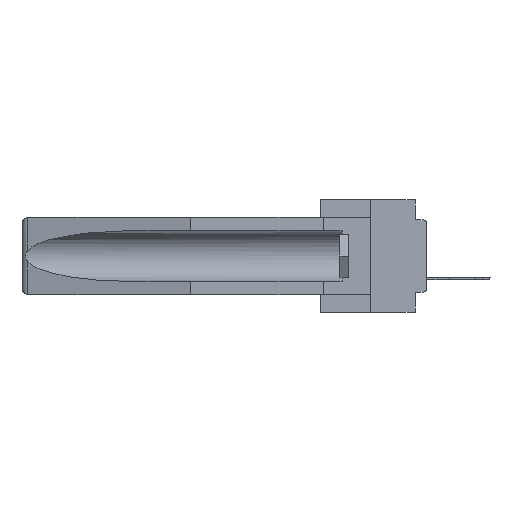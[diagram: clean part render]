
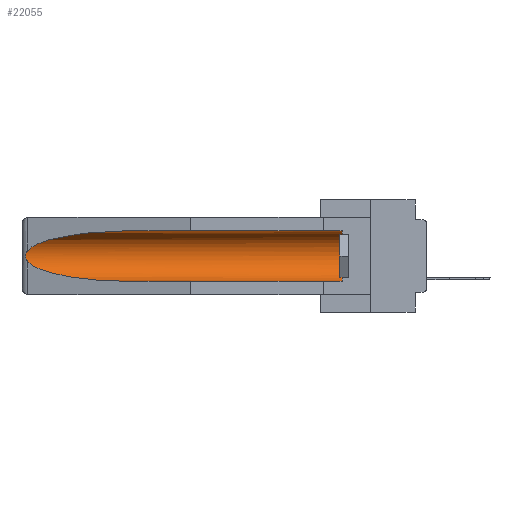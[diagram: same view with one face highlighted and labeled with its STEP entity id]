
A CAD part, left-side view. The second image highlights one B-rep face of the part: STEP entity #22055.
In plain terms, the highlighted cylindrical face has radius 2.857 mm (diameter 5.715 mm), a partial arc.
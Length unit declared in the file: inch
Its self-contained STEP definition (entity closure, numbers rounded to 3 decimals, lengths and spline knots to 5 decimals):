
#254 = CARTESIAN_POINT ( 'NONE',  ( 0.2673, 1.53269, -0.17917 ) ) ;
#654 = CARTESIAN_POINT ( 'NONE',  ( 0.155, 0.126, -0.1715 ) ) ;
#668 = CARTESIAN_POINT ( 'NONE',  ( 0.26537, 1.52718, -0.14972 ) ) ;
#1073 = ORIENTED_EDGE ( 'NONE', *, *, #18933, .F. ) ;
#1545 = LINE ( 'NONE', #14667, #8756 ) ;
#1700 = DIRECTION ( 'NONE',  ( 0., 1., 0. ) ) ;
#3246 = CARTESIAN_POINT ( 'NONE',  ( 0.155, -0.30754, -0.284 ) ) ;
#3362 = FACE_OUTER_BOUND ( 'NONE', #4756, .T. ) ;
#4249 = CARTESIAN_POINT ( 'NONE',  ( 0.26655, 1.53094, -0.18657 ) ) ;
#4392 = CARTESIAN_POINT ( 'NONE',  ( 0.26654, 1.53092, -0.15636 ) ) ;
#4756 = EDGE_LOOP ( 'NONE', ( #9486, #28176, #26582, #1073, #17301, #28006 ) ) ;
#4899 = EDGE_CURVE ( 'NONE', #9115, #27358, #9374, .T. ) ;
#4945 = EDGE_CURVE ( 'NONE', #11408, #9115, #16770, .T. ) ;
#6420 = DIRECTION ( 'NONE',  ( 0., 0., 1. ) ) ;
#7670 = LINE ( 'NONE', #3246, #9727 ) ;
#7814 = DIRECTION ( 'NONE',  ( 0., 1., 0. ) ) ;
#8195 = VERTEX_POINT ( 'NONE', #13341 ) ;
#8678 = CARTESIAN_POINT ( 'NONE',  ( 0.26597, 1.52961, -0.15275 ) ) ;
#8756 = VECTOR ( 'NONE', #1700, 39.37008 ) ;
#8793 = EDGE_CURVE ( 'NONE', #8195, #11408, #1545, .T. ) ;
#8954 = CARTESIAN_POINT ( 'NONE',  ( 0.26537, 1.52718, -0.19328 ) ) ;
#9115 = VERTEX_POINT ( 'NONE', #9651 ) ;
#9374 = B_SPLINE_CURVE_WITH_KNOTS ( 'NONE', 3,
 ( #15514, #8678, #4392, #17663, #15385, #15655, #254, #4249, #11243, #8954 ),
 .UNSPECIFIED., .F., .F.,
 ( 4, 2, 2, 2, 4 ),
 ( 0., 0.00029, 0.00058, 0.00087, 0.00117 ),
 .UNSPECIFIED. ) ;
#9486 = ORIENTED_EDGE ( 'NONE', *, *, #4945, .T. ) ;
#9496 = DIRECTION ( 'NONE',  ( 0., -1., 0. ) ) ;
#9651 = CARTESIAN_POINT ( 'NONE',  ( 0.26537, 1.52718, -0.14972 ) ) ;
#9652 = CARTESIAN_POINT ( 'NONE',  ( 0.155, -0.30754, -0.1715 ) ) ;
#9727 = VECTOR ( 'NONE', #7814, 39.37008 ) ;
#11243 = CARTESIAN_POINT ( 'NONE',  ( 0.26597, 1.5296, -0.19026 ) ) ;
#11408 = VERTEX_POINT ( 'NONE', #16053 ) ;
#11483 = EDGE_CURVE ( 'NONE', #27839, #8195, #13899, .T. ) ;
#11609 = CARTESIAN_POINT ( 'NONE',  ( 0.155, 0.126, -0.284 ) ) ;
#12072 = DIRECTION ( 'NONE',  ( 0., 1., 0. ) ) ;
#12428 = CARTESIAN_POINT ( 'NONE',  ( 0.26537, 1.52718, -0.19328 ) ) ;
#13341 = CARTESIAN_POINT ( 'NONE',  ( 0.155, 0.126, -0.059 ) ) ;
#13457 = AXIS2_PLACEMENT_3D ( 'NONE', #9652, #12072, #20755 ) ;
#13861 = CARTESIAN_POINT ( 'NONE',  ( 0.155, 1.07973, -0.284 ) ) ;
#13899 = CIRCLE ( 'NONE', #27975, 0.1125 ) ;
#14030 =( BOUNDED_CURVE ( )  B_SPLINE_CURVE ( 3, ( #26724, #21908, #17021, #15174 ),
 .UNSPECIFIED., .F., .F. ) 
 B_SPLINE_CURVE_WITH_KNOTS ( ( 4, 4 ),
 ( 0.1948, 1.5708 ),
 .UNSPECIFIED. ) 
 CURVE ( )  GEOMETRIC_REPRESENTATION_ITEM ( )  RATIONAL_B_SPLINE_CURVE ( ( 1., 0.848, 0.848, 1. ) ) 
 REPRESENTATION_ITEM ( '' )  );
#14070 = CARTESIAN_POINT ( 'NONE',  ( 0.155, 1.07973, -0.059 ) ) ;
#14667 = CARTESIAN_POINT ( 'NONE',  ( 0.155, -0.30754, -0.059 ) ) ;
#15174 = CARTESIAN_POINT ( 'NONE',  ( 0.155, 1.07973, -0.284 ) ) ;
#15385 = CARTESIAN_POINT ( 'NONE',  ( 0.2675, 1.53308, -0.16763 ) ) ;
#15514 = CARTESIAN_POINT ( 'NONE',  ( 0.26537, 1.52718, -0.14972 ) ) ;
#15655 = CARTESIAN_POINT ( 'NONE',  ( 0.2675, 1.53308, -0.17534 ) ) ;
#16053 = CARTESIAN_POINT ( 'NONE',  ( 0.155, 1.07973, -0.059 ) ) ;
#16770 =( BOUNDED_CURVE ( )  B_SPLINE_CURVE ( 3, ( #14070, #22329, #18074, #668 ),
 .UNSPECIFIED., .F., .F. ) 
 B_SPLINE_CURVE_WITH_KNOTS ( ( 4, 4 ),
 ( 4.71239, 6.08839 ),
 .UNSPECIFIED. ) 
 CURVE ( )  GEOMETRIC_REPRESENTATION_ITEM ( )  RATIONAL_B_SPLINE_CURVE ( ( 1., 0.848, 0.848, 1. ) ) 
 REPRESENTATION_ITEM ( '' )  );
#17021 = CARTESIAN_POINT ( 'NONE',  ( 0.21114, 1.30732, -0.284 ) ) ;
#17301 = ORIENTED_EDGE ( 'NONE', *, *, #11483, .T. ) ;
#17663 = CARTESIAN_POINT ( 'NONE',  ( 0.2673, 1.5327, -0.16383 ) ) ;
#18074 = CARTESIAN_POINT ( 'NONE',  ( 0.25451, 1.48313, -0.09465 ) ) ;
#18623 = CYLINDRICAL_SURFACE ( 'NONE', #13457, 0.1125 ) ;
#18933 = EDGE_CURVE ( 'NONE', #27839, #27212, #7670, .T. ) ;
#20755 = DIRECTION ( 'NONE',  ( 0., 0., 1. ) ) ;
#21908 = CARTESIAN_POINT ( 'NONE',  ( 0.25451, 1.48313, -0.24835 ) ) ;
#22055 = ADVANCED_FACE ( 'NONE', ( #3362 ), #18623, .F. ) ;
#22329 = CARTESIAN_POINT ( 'NONE',  ( 0.21114, 1.30732, -0.059 ) ) ;
#26582 = ORIENTED_EDGE ( 'NONE', *, *, #26873, .T. ) ;
#26724 = CARTESIAN_POINT ( 'NONE',  ( 0.26537, 1.52718, -0.19328 ) ) ;
#26873 = EDGE_CURVE ( 'NONE', #27358, #27212, #14030, .T. ) ;
#27212 = VERTEX_POINT ( 'NONE', #13861 ) ;
#27358 = VERTEX_POINT ( 'NONE', #12428 ) ;
#27839 = VERTEX_POINT ( 'NONE', #11609 ) ;
#27975 = AXIS2_PLACEMENT_3D ( 'NONE', #654, #9496, #6420 ) ;
#28006 = ORIENTED_EDGE ( 'NONE', *, *, #8793, .T. ) ;
#28176 = ORIENTED_EDGE ( 'NONE', *, *, #4899, .T. ) ;
